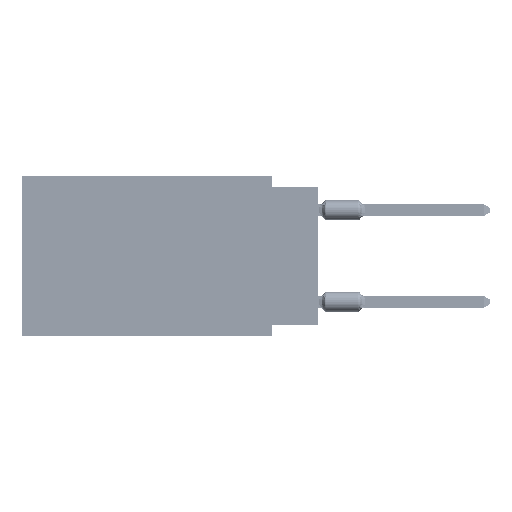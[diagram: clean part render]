
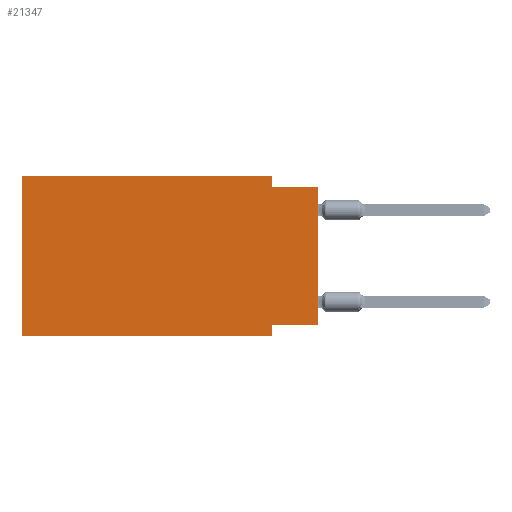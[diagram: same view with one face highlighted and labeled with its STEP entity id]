
A CAD part, left-side view. The second image highlights one B-rep face of the part: STEP entity #21347.
In plain terms, the highlighted planar face has unit normal (-1, 0, 0).
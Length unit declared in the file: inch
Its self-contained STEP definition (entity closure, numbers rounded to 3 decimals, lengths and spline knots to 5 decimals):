
#4281 = DIRECTION ( 'NONE',  ( 0., 1., 0. ) ) ;
#5797 = EDGE_LOOP ( 'NONE', ( #68998, #5960, #51981, #116728, #29869, #14762, #8718, #39196 ) ) ;
#5960 = ORIENTED_EDGE ( 'NONE', *, *, #29548, .F. ) ;
#7868 = VECTOR ( 'NONE', #88413, 39.37008 ) ;
#8243 = EDGE_CURVE ( 'NONE', #59706, #86582, #37138, .T. ) ;
#8718 = ORIENTED_EDGE ( 'NONE', *, *, #75364, .F. ) ;
#9740 = CARTESIAN_POINT ( 'NONE',  ( 0., 0.1, 0. ) ) ;
#9841 = VERTEX_POINT ( 'NONE', #18398 ) ;
#10717 = CARTESIAN_POINT ( 'NONE',  ( 0., 0.645, 0. ) ) ;
#13562 = CARTESIAN_POINT ( 'NONE',  ( 0., 0.1, -0.35 ) ) ;
#14762 = ORIENTED_EDGE ( 'NONE', *, *, #108782, .T. ) ;
#15350 = CARTESIAN_POINT ( 'NONE',  ( 0., 0.1, 0. ) ) ;
#18098 = CARTESIAN_POINT ( 'NONE',  ( 0., 0.645, -0.35 ) ) ;
#18398 = CARTESIAN_POINT ( 'NONE',  ( 0., 0., -0.025 ) ) ;
#18561 = CARTESIAN_POINT ( 'NONE',  ( 0., 0., -0.325 ) ) ;
#19897 = CARTESIAN_POINT ( 'NONE',  ( 0., 0., -0.325 ) ) ;
#20014 = AXIS2_PLACEMENT_3D ( 'NONE', #69890, #106511, #60913 ) ;
#21347 = ADVANCED_FACE ( 'NONE', ( #78882 ), #33243, .F. ) ;
#26124 = DIRECTION ( 'NONE',  ( 0., 0., 1. ) ) ;
#27101 = LINE ( 'NONE', #18098, #7868 ) ;
#29548 = EDGE_CURVE ( 'NONE', #30330, #9841, #82076, .T. ) ;
#29869 = ORIENTED_EDGE ( 'NONE', *, *, #48820, .F. ) ;
#30330 = VERTEX_POINT ( 'NONE', #99221 ) ;
#30486 = LINE ( 'NONE', #106083, #109616 ) ;
#33243 = PLANE ( 'NONE',  #20014 ) ;
#34559 = DIRECTION ( 'NONE',  ( 0., 0., -1. ) ) ;
#35120 = LINE ( 'NONE', #108364, #45576 ) ;
#35125 = VERTEX_POINT ( 'NONE', #81342 ) ;
#35234 = EDGE_CURVE ( 'NONE', #63252, #9841, #35120, .T. ) ;
#37138 = LINE ( 'NONE', #10717, #65704 ) ;
#38535 = LINE ( 'NONE', #19897, #62794 ) ;
#39196 = ORIENTED_EDGE ( 'NONE', *, *, #41300, .F. ) ;
#41300 = EDGE_CURVE ( 'NONE', #63252, #35125, #38535, .T. ) ;
#44337 = VERTEX_POINT ( 'NONE', #113813 ) ;
#45576 = VECTOR ( 'NONE', #26124, 39.37008 ) ;
#45612 = EDGE_CURVE ( 'NONE', #86582, #30330, #96417, .T. ) ;
#47365 = DIRECTION ( 'NONE',  ( 0., -1., 0. ) ) ;
#48283 = VECTOR ( 'NONE', #68215, 39.37008 ) ;
#48820 = EDGE_CURVE ( 'NONE', #83163, #59706, #30486, .T. ) ;
#49828 = CARTESIAN_POINT ( 'NONE',  ( 0., 0.645, -0.35 ) ) ;
#49947 = VECTOR ( 'NONE', #34559, 39.37008 ) ;
#51981 = ORIENTED_EDGE ( 'NONE', *, *, #45612, .F. ) ;
#59352 = VECTOR ( 'NONE', #116486, 39.37008 ) ;
#59706 = VERTEX_POINT ( 'NONE', #71135 ) ;
#60913 = DIRECTION ( 'NONE',  ( 0., 0., -1. ) ) ;
#62794 = VECTOR ( 'NONE', #4281, 39.37008 ) ;
#63252 = VERTEX_POINT ( 'NONE', #18561 ) ;
#65704 = VECTOR ( 'NONE', #47365, 39.37008 ) ;
#68215 = DIRECTION ( 'NONE',  ( 0., 0., -1. ) ) ;
#68998 = ORIENTED_EDGE ( 'NONE', *, *, #35234, .T. ) ;
#69890 = CARTESIAN_POINT ( 'NONE',  ( 0., 0.645, 0. ) ) ;
#71135 = CARTESIAN_POINT ( 'NONE',  ( 0., 0.645, 0. ) ) ;
#75364 = EDGE_CURVE ( 'NONE', #35125, #44337, #113818, .T. ) ;
#78882 = FACE_OUTER_BOUND ( 'NONE', #5797, .T. ) ;
#81342 = CARTESIAN_POINT ( 'NONE',  ( 0., 0.1, -0.325 ) ) ;
#82076 = LINE ( 'NONE', #97877, #59352 ) ;
#83163 = VERTEX_POINT ( 'NONE', #49828 ) ;
#86582 = VERTEX_POINT ( 'NONE', #9740 ) ;
#88413 = DIRECTION ( 'NONE',  ( 0., -1., 0. ) ) ;
#96417 = LINE ( 'NONE', #15350, #49947 ) ;
#97877 = CARTESIAN_POINT ( 'NONE',  ( 0., 0., -0.025 ) ) ;
#99221 = CARTESIAN_POINT ( 'NONE',  ( 0., 0.1, -0.025 ) ) ;
#103704 = DIRECTION ( 'NONE',  ( 0., 0., 1. ) ) ;
#106083 = CARTESIAN_POINT ( 'NONE',  ( 0., 0.645, 0. ) ) ;
#106511 = DIRECTION ( 'NONE',  ( 1., 0., 0. ) ) ;
#108364 = CARTESIAN_POINT ( 'NONE',  ( 0., 0., 0. ) ) ;
#108782 = EDGE_CURVE ( 'NONE', #83163, #44337, #27101, .T. ) ;
#109616 = VECTOR ( 'NONE', #103704, 39.37008 ) ;
#113813 = CARTESIAN_POINT ( 'NONE',  ( 0., 0.1, -0.35 ) ) ;
#113818 = LINE ( 'NONE', #13562, #48283 ) ;
#116486 = DIRECTION ( 'NONE',  ( 0., -1., 0. ) ) ;
#116728 = ORIENTED_EDGE ( 'NONE', *, *, #8243, .F. ) ;
